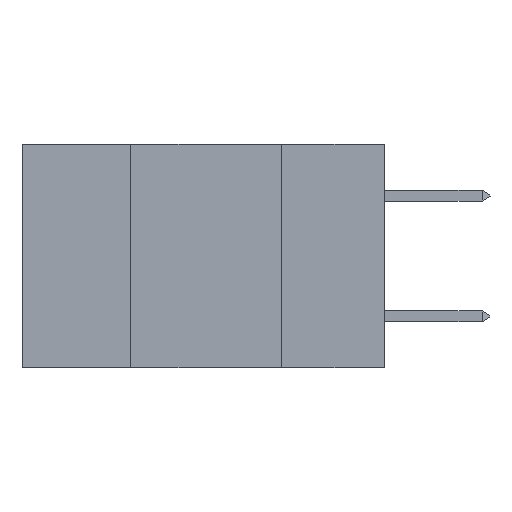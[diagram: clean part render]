
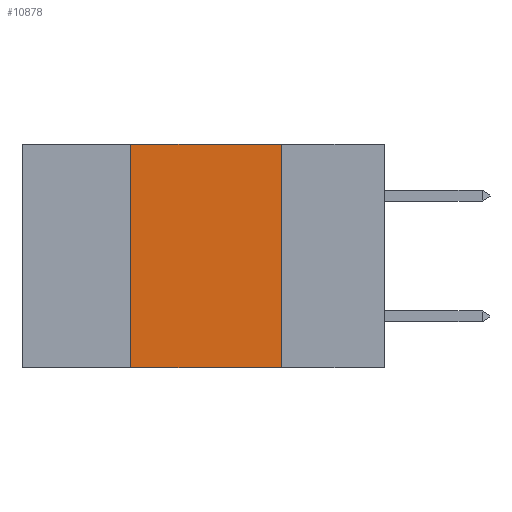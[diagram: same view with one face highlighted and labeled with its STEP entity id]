
A CAD part, left-side view. The second image highlights one B-rep face of the part: STEP entity #10878.
In plain terms, the highlighted planar face has unit normal (-1, 0, 0).
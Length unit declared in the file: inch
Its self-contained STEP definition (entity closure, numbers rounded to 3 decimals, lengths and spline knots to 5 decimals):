
#555 = CARTESIAN_POINT ( 'NONE',  ( 0., 0.17, -0.37 ) ) ;
#606 = CARTESIAN_POINT ( 'NONE',  ( 0., 0.6, 0. ) ) ;
#1854 = FACE_OUTER_BOUND ( 'NONE', #12494, .T. ) ;
#2874 = LINE ( 'NONE', #6405, #3723 ) ;
#3149 = LINE ( 'NONE', #9240, #20157 ) ;
#3723 = VECTOR ( 'NONE', #26678, 39.37008 ) ;
#4079 = VERTEX_POINT ( 'NONE', #555 ) ;
#6405 = CARTESIAN_POINT ( 'NONE',  ( 0., 0.42, 0. ) ) ;
#6696 = DIRECTION ( 'NONE',  ( 0., 0., -1. ) ) ;
#6885 = DIRECTION ( 'NONE',  ( 0., -1., 0. ) ) ;
#7409 = DIRECTION ( 'NONE',  ( 0., -1., 0. ) ) ;
#7919 = VECTOR ( 'NONE', #7409, 39.37008 ) ;
#9080 = VERTEX_POINT ( 'NONE', #19516 ) ;
#9240 = CARTESIAN_POINT ( 'NONE',  ( 0., 0.17, 0. ) ) ;
#9359 = EDGE_CURVE ( 'NONE', #14012, #33797, #30304, .T. ) ;
#9722 = ORIENTED_EDGE ( 'NONE', *, *, #36074, .F. ) ;
#10111 = ORIENTED_EDGE ( 'NONE', *, *, #9359, .F. ) ;
#10878 = ADVANCED_FACE ( 'NONE', ( #1854 ), #17177, .F. ) ;
#12494 = EDGE_LOOP ( 'NONE', ( #9722, #10111, #23126, #17611 ) ) ;
#14012 = VERTEX_POINT ( 'NONE', #19730 ) ;
#14391 = DIRECTION ( 'NONE',  ( 0., 0., -1. ) ) ;
#15981 = CARTESIAN_POINT ( 'NONE',  ( 0., 0.17, 0. ) ) ;
#16846 = CARTESIAN_POINT ( 'NONE',  ( 0., 0.6, -0.37 ) ) ;
#17177 = PLANE ( 'NONE',  #20403 ) ;
#17611 = ORIENTED_EDGE ( 'NONE', *, *, #23320, .T. ) ;
#19516 = CARTESIAN_POINT ( 'NONE',  ( 0., 0.42, -0.37 ) ) ;
#19730 = CARTESIAN_POINT ( 'NONE',  ( 0., 0.42, 0. ) ) ;
#20157 = VECTOR ( 'NONE', #6696, 39.37008 ) ;
#20403 = AXIS2_PLACEMENT_3D ( 'NONE', #29173, #29366, #14391 ) ;
#21888 = VECTOR ( 'NONE', #6885, 39.37008 ) ;
#23126 = ORIENTED_EDGE ( 'NONE', *, *, #31886, .F. ) ;
#23320 = EDGE_CURVE ( 'NONE', #9080, #4079, #25533, .T. ) ;
#25533 = LINE ( 'NONE', #16846, #7919 ) ;
#26678 = DIRECTION ( 'NONE',  ( 0., 0., 1. ) ) ;
#29173 = CARTESIAN_POINT ( 'NONE',  ( 0., 0.6, 0. ) ) ;
#29366 = DIRECTION ( 'NONE',  ( 1., 0., 0. ) ) ;
#30304 = LINE ( 'NONE', #606, #21888 ) ;
#31886 = EDGE_CURVE ( 'NONE', #9080, #14012, #2874, .T. ) ;
#33797 = VERTEX_POINT ( 'NONE', #15981 ) ;
#36074 = EDGE_CURVE ( 'NONE', #33797, #4079, #3149, .T. ) ;
